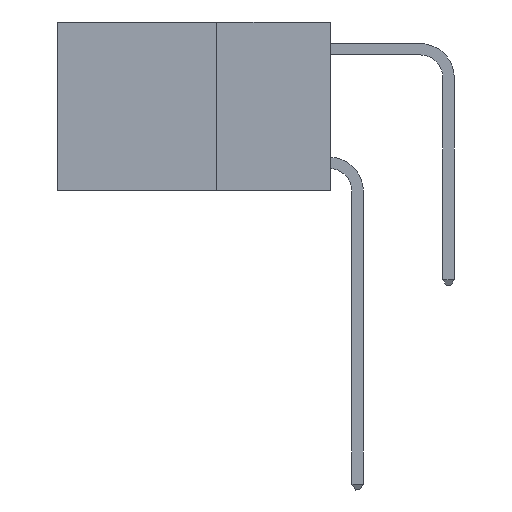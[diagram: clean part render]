
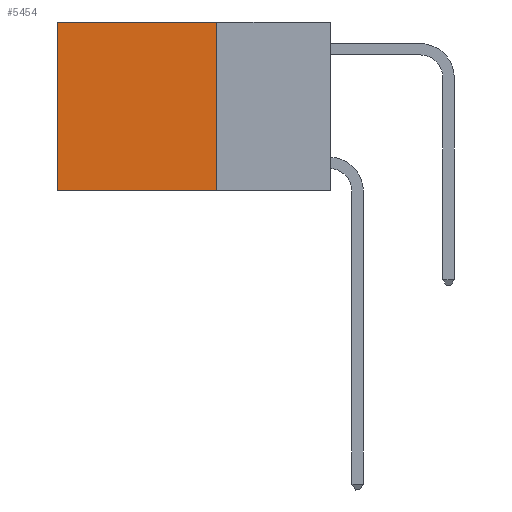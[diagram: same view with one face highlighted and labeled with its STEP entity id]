
A CAD part, left-side view. The second image highlights one B-rep face of the part: STEP entity #5454.
In plain terms, the highlighted planar face has unit normal (-1, 0, 0).
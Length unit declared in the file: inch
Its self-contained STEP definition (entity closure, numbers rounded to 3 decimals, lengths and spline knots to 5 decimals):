
#534 = VERTEX_POINT ( 'NONE', #12073 ) ;
#694 = CARTESIAN_POINT ( 'NONE',  ( 0.2625, 0.25, 0. ) ) ;
#1560 = VECTOR ( 'NONE', #13441, 39.37008 ) ;
#1694 = VECTOR ( 'NONE', #8782, 39.37008 ) ;
#1902 = LINE ( 'NONE', #10350, #14496 ) ;
#1916 = VERTEX_POINT ( 'NONE', #2909 ) ;
#2909 = CARTESIAN_POINT ( 'NONE',  ( 0.2625, 0.6, -0.37 ) ) ;
#3452 = CARTESIAN_POINT ( 'NONE',  ( 0.2625, 0.25, -0.37 ) ) ;
#3564 = ORIENTED_EDGE ( 'NONE', *, *, #5821, .F. ) ;
#3796 = ORIENTED_EDGE ( 'NONE', *, *, #12650, .T. ) ;
#4401 = EDGE_CURVE ( 'NONE', #534, #1916, #14119, .T. ) ;
#5454 = ADVANCED_FACE ( 'NONE', ( #9103 ), #14258, .F. ) ;
#5821 = EDGE_CURVE ( 'NONE', #10344, #1916, #11026, .T. ) ;
#7206 = VERTEX_POINT ( 'NONE', #694 ) ;
#7210 = EDGE_LOOP ( 'NONE', ( #12739, #3564, #15125, #3796 ) ) ;
#7353 = CARTESIAN_POINT ( 'NONE',  ( 0.2625, 0.6, 0. ) ) ;
#8152 = DIRECTION ( 'NONE',  ( 0., 0., -1. ) ) ;
#8373 = EDGE_CURVE ( 'NONE', #7206, #10344, #11346, .T. ) ;
#8782 = DIRECTION ( 'NONE',  ( 0., 1., 0. ) ) ;
#9103 = FACE_OUTER_BOUND ( 'NONE', #7210, .T. ) ;
#10295 = AXIS2_PLACEMENT_3D ( 'NONE', #11802, #15490, #8152 ) ;
#10324 = DIRECTION ( 'NONE',  ( 0., 0., -1. ) ) ;
#10344 = VERTEX_POINT ( 'NONE', #3452 ) ;
#10350 = CARTESIAN_POINT ( 'NONE',  ( 0.2625, 0.25, 0. ) ) ;
#10971 = VECTOR ( 'NONE', #10324, 39.37008 ) ;
#11026 = LINE ( 'NONE', #12432, #1694 ) ;
#11346 = LINE ( 'NONE', #13950, #10971 ) ;
#11802 = CARTESIAN_POINT ( 'NONE',  ( 0.2625, 0.25, 0. ) ) ;
#12073 = CARTESIAN_POINT ( 'NONE',  ( 0.2625, 0.6, 0. ) ) ;
#12432 = CARTESIAN_POINT ( 'NONE',  ( 0.2625, 0.25, -0.37 ) ) ;
#12650 = EDGE_CURVE ( 'NONE', #7206, #534, #1902, .T. ) ;
#12739 = ORIENTED_EDGE ( 'NONE', *, *, #4401, .T. ) ;
#13441 = DIRECTION ( 'NONE',  ( 0., 0., -1. ) ) ;
#13950 = CARTESIAN_POINT ( 'NONE',  ( 0.2625, 0.25, 0. ) ) ;
#14119 = LINE ( 'NONE', #7353, #1560 ) ;
#14258 = PLANE ( 'NONE',  #10295 ) ;
#14496 = VECTOR ( 'NONE', #15269, 39.37008 ) ;
#15125 = ORIENTED_EDGE ( 'NONE', *, *, #8373, .F. ) ;
#15269 = DIRECTION ( 'NONE',  ( 0., 1., 0. ) ) ;
#15490 = DIRECTION ( 'NONE',  ( 1., 0., 0. ) ) ;
